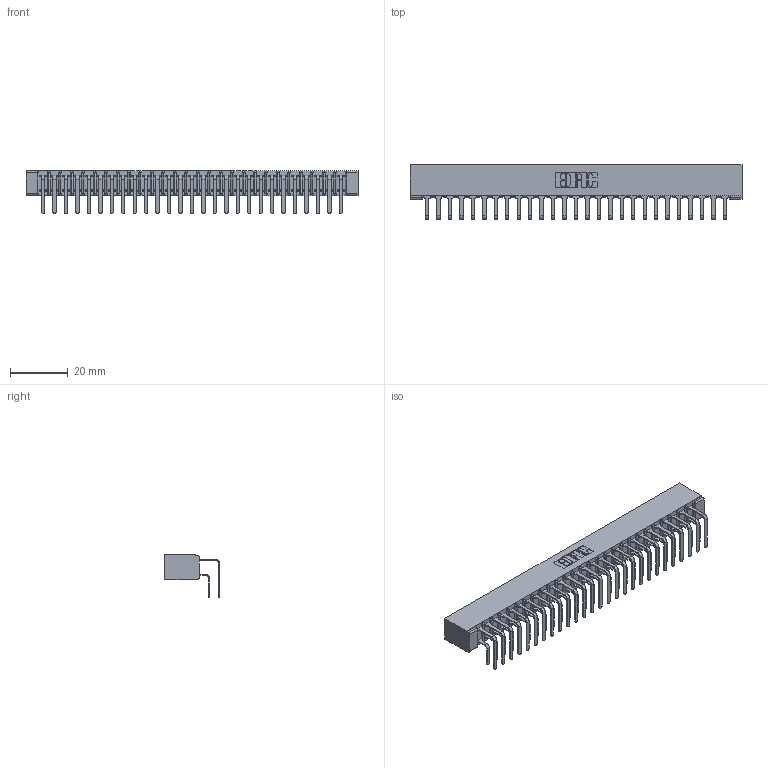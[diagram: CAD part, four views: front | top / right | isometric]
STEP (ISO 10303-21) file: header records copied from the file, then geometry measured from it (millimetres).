
FILE_DESCRIPTION (( 'STEP AP203' ), '1' );
FILE_NAME ('357-054-558-201.STEP', '2019-09-19T04:13:36', ( '' ), ( '' ), 'SwSTEP 2.0', 'SolidWorks 2016', '' );
FILE_SCHEMA (( 'CONFIG_CONTROL_DESIGN' ));
Length unit declared in the file: inch
Products named in the file (4): 357-054-558-201; 307-290-001_558 559 - 1 (Single); 307 Part_No Mounting Lugs; 307-290-001_558 - 2 (Single)
Assembly tree (55 placements, depth 2):
  357-054-558-201
    307 Part_No Mounting Lugs
    307-290-001_558 559 - 1 (Single)  x27
    307-290-001_558 - 2 (Single)  x27
Bounding box: 114.86 x 18.96 x 14.81 mm (x, y, z)
Volume: 7984.9 mm3; surface area: 16182.4 mm2
Topology: 55 solids, 55 shells, 2838 faces, 7967 edges, 5162 vertices
Faces by surface type: plane 1848, cylinder 934, sphere 56
Entity records: 27029 total; most frequent: CARTESIAN_POINT 4425, ORIENTED_EDGE 4382, DIRECTION 4339, EDGE_CURVE 2191, VECTOR 1675, LINE 1675, VERTEX_POINT 1418, AXIS2_PLACEMENT_3D 1332
